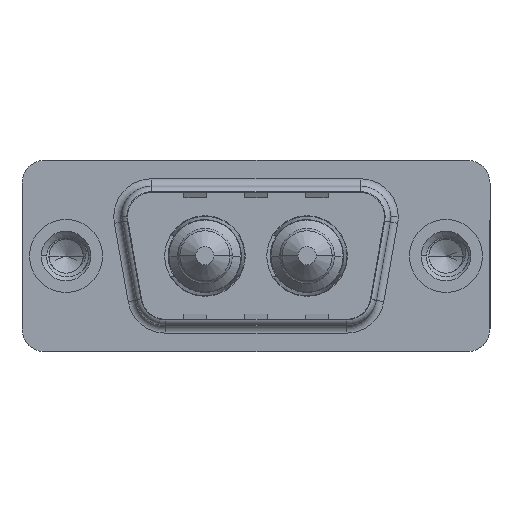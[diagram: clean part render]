
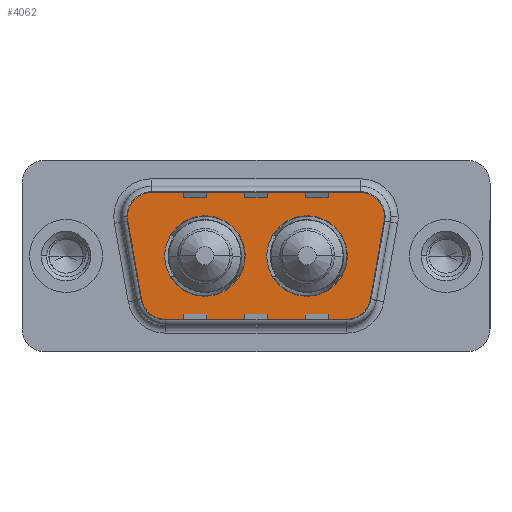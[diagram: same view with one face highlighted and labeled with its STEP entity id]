
A CAD part, top view. The second image highlights one B-rep face of the part: STEP entity #4062.
In plain terms, the highlighted planar face has unit normal (0, 0, 1).
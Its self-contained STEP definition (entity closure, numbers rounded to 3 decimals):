
#124 = DIRECTION ( 'NONE',  ( 0., 0., 1. ) ) ;
#154 = CARTESIAN_POINT ( 'NONE',  ( 4.489, -3.247, 0. ) ) ;
#207 = CARTESIAN_POINT ( 'NONE',  ( 5.436, 2.9, 0. ) ) ;
#245 = CIRCLE ( 'NONE', #4522, 2.65 ) ;
#307 = DIRECTION ( 'NONE',  ( 0., 0., 1. ) ) ;
#355 = DIRECTION ( 'NONE',  ( 0., 0., 1. ) ) ;
#426 = DIRECTION ( 'NONE',  ( -1., 0., 0. ) ) ;
#441 = DIRECTION ( 'NONE',  ( 0., 0., 1. ) ) ;
#458 = CARTESIAN_POINT ( 'NONE',  ( 9.14, 0., 0. ) ) ;
#484 = DIRECTION ( 'NONE',  ( 1., 0., 0. ) ) ;
#499 = DIRECTION ( 'NONE',  ( 1., 0., 0. ) ) ;
#538 = CARTESIAN_POINT ( 'NONE',  ( 3.466, 2.553, 0. ) ) ;
#560 = EDGE_CURVE ( 'NONE', #12153, #6827, #3407, .T. ) ;
#587 = CARTESIAN_POINT ( 'NONE',  ( 18.541, -4.9, 0. ) ) ;
#664 = DIRECTION ( 'NONE',  ( 0., 0., 1. ) ) ;
#837 = VERTEX_POINT ( 'NONE', #5940 ) ;
#878 = EDGE_CURVE ( 'NONE', #1156, #8185, #3256, .T. ) ;
#952 = EDGE_CURVE ( 'NONE', #6827, #12153, #5564, .T. ) ;
#1031 = LINE ( 'NONE', #9807, #10657 ) ;
#1056 = CARTESIAN_POINT ( 'NONE',  ( 15.86, 0., 0. ) ) ;
#1123 = VECTOR ( 'NONE', #4236, 1000. ) ;
#1156 = VERTEX_POINT ( 'NONE', #9752 ) ;
#1205 = DIRECTION ( 'NONE',  ( 1., 0., 0. ) ) ;
#1322 = ORIENTED_EDGE ( 'NONE', *, *, #3347, .F. ) ;
#1721 = LINE ( 'NONE', #3648, #1123 ) ;
#1875 = CARTESIAN_POINT ( 'NONE',  ( 18.541, -2.9, 0. ) ) ;
#1966 = ORIENTED_EDGE ( 'NONE', *, *, #2773, .T. ) ;
#2060 = EDGE_CURVE ( 'NONE', #8839, #4864, #4943, .T. ) ;
#2067 = DIRECTION ( 'NONE',  ( 1., 0., 0. ) ) ;
#2173 = FACE_BOUND ( 'NONE', #10236, .T. ) ;
#2336 = CIRCLE ( 'NONE', #7982, 2. ) ;
#2423 = VERTEX_POINT ( 'NONE', #6713 ) ;
#2604 = CARTESIAN_POINT ( 'NONE',  ( 6.459, -4.9, 0. ) ) ;
#2773 = EDGE_CURVE ( 'NONE', #5269, #12408, #7639, .T. ) ;
#2802 = ORIENTED_EDGE ( 'NONE', *, *, #5728, .T. ) ;
#2943 = AXIS2_PLACEMENT_3D ( 'NONE', #207, #441, #1205 ) ;
#3172 = EDGE_CURVE ( 'NONE', #5515, #2423, #2336, .T. ) ;
#3201 = DIRECTION ( 'NONE',  ( 1., 0., 0. ) ) ;
#3256 = CIRCLE ( 'NONE', #4818, 2. ) ;
#3347 = EDGE_CURVE ( 'NONE', #4761, #837, #245, .T. ) ;
#3407 = CIRCLE ( 'NONE', #5064, 2.65 ) ;
#3524 = AXIS2_PLACEMENT_3D ( 'NONE', #5838, #6750, #12303 ) ;
#3648 = CARTESIAN_POINT ( 'NONE',  ( 5.436, 4.9, 0. ) ) ;
#3705 = CARTESIAN_POINT ( 'NONE',  ( 6.459, -4.9, 0. ) ) ;
#3807 = LINE ( 'NONE', #5099, #5806 ) ;
#3814 = EDGE_CURVE ( 'NONE', #8185, #8839, #1721, .T. ) ;
#3886 = ORIENTED_EDGE ( 'NONE', *, *, #7821, .F. ) ;
#4062 = ADVANCED_FACE ( 'NONE', ( #4433, #2173, #6999 ), #6390, .T. ) ;
#4107 = ORIENTED_EDGE ( 'NONE', *, *, #3814, .T. ) ;
#4236 = DIRECTION ( 'NONE',  ( -1., 0., 0. ) ) ;
#4362 = CARTESIAN_POINT ( 'NONE',  ( 18.51, 0., 0. ) ) ;
#4433 = FACE_BOUND ( 'NONE', #10389, .T. ) ;
#4522 = AXIS2_PLACEMENT_3D ( 'NONE', #458, #355, #484 ) ;
#4574 = DIRECTION ( 'NONE',  ( 0.174, 0.985, 0. ) ) ;
#4695 = AXIS2_PLACEMENT_3D ( 'NONE', #1875, #664, #499 ) ;
#4761 = VERTEX_POINT ( 'NONE', #9322 ) ;
#4818 = AXIS2_PLACEMENT_3D ( 'NONE', #12176, #5378, #426 ) ;
#4864 = VERTEX_POINT ( 'NONE', #538 ) ;
#4943 = CIRCLE ( 'NONE', #2943, 2. ) ;
#5064 = AXIS2_PLACEMENT_3D ( 'NONE', #11351, #11273, #9793 ) ;
#5099 = CARTESIAN_POINT ( 'NONE',  ( 3.466, 2.553, 0. ) ) ;
#5269 = VERTEX_POINT ( 'NONE', #154 ) ;
#5378 = DIRECTION ( 'NONE',  ( 0., 0., 1. ) ) ;
#5380 = EDGE_CURVE ( 'NONE', #12408, #5515, #6913, .T. ) ;
#5515 = VERTEX_POINT ( 'NONE', #587 ) ;
#5564 = CIRCLE ( 'NONE', #7404, 2.65 ) ;
#5728 = EDGE_CURVE ( 'NONE', #2423, #7436, #1031, .T. ) ;
#5754 = CARTESIAN_POINT ( 'NONE',  ( 19.564, 4.9, 0. ) ) ;
#5806 = VECTOR ( 'NONE', #6979, 1000. ) ;
#5838 = CARTESIAN_POINT ( 'NONE',  ( 6.459, -2.9, 0. ) ) ;
#5900 = CARTESIAN_POINT ( 'NONE',  ( 19.564, 2.9, 0. ) ) ;
#5940 = CARTESIAN_POINT ( 'NONE',  ( 6.49, 0., 0. ) ) ;
#5942 = DIRECTION ( 'NONE',  ( 0., 0., 1. ) ) ;
#5987 = CARTESIAN_POINT ( 'NONE',  ( 13.21, 0., 0. ) ) ;
#6082 = CARTESIAN_POINT ( 'NONE',  ( 9.14, 0., 0. ) ) ;
#6390 = PLANE ( 'NONE',  #4695 ) ;
#6405 = CIRCLE ( 'NONE', #12018, 2. ) ;
#6713 = CARTESIAN_POINT ( 'NONE',  ( 20.511, -3.247, 0. ) ) ;
#6750 = DIRECTION ( 'NONE',  ( 0., 0., 1. ) ) ;
#6827 = VERTEX_POINT ( 'NONE', #5987 ) ;
#6842 = CARTESIAN_POINT ( 'NONE',  ( 5.436, 4.9, 0. ) ) ;
#6847 = DIRECTION ( 'NONE',  ( -1., 0., 0. ) ) ;
#6913 = LINE ( 'NONE', #2604, #9761 ) ;
#6979 = DIRECTION ( 'NONE',  ( 0.174, -0.985, 0. ) ) ;
#6999 = FACE_OUTER_BOUND ( 'NONE', #10603, .T. ) ;
#7042 = DIRECTION ( 'NONE',  ( 1., 0., 0. ) ) ;
#7235 = EDGE_CURVE ( 'NONE', #7436, #1156, #6405, .T. ) ;
#7404 = AXIS2_PLACEMENT_3D ( 'NONE', #1056, #8881, #2067 ) ;
#7436 = VERTEX_POINT ( 'NONE', #12067 ) ;
#7553 = ORIENTED_EDGE ( 'NONE', *, *, #3172, .T. ) ;
#7639 = CIRCLE ( 'NONE', #3524, 2. ) ;
#7821 = EDGE_CURVE ( 'NONE', #837, #4761, #8658, .T. ) ;
#7982 = AXIS2_PLACEMENT_3D ( 'NONE', #10172, #5942, #9683 ) ;
#8095 = ORIENTED_EDGE ( 'NONE', *, *, #7235, .T. ) ;
#8185 = VERTEX_POINT ( 'NONE', #5754 ) ;
#8316 = EDGE_CURVE ( 'NONE', #4864, #5269, #3807, .T. ) ;
#8658 = CIRCLE ( 'NONE', #11537, 2.65 ) ;
#8839 = VERTEX_POINT ( 'NONE', #6842 ) ;
#8881 = DIRECTION ( 'NONE',  ( 0., 0., 1. ) ) ;
#9286 = ORIENTED_EDGE ( 'NONE', *, *, #878, .T. ) ;
#9322 = CARTESIAN_POINT ( 'NONE',  ( 11.79, 0., 0. ) ) ;
#9683 = DIRECTION ( 'NONE',  ( 1., 0., 0. ) ) ;
#9752 = CARTESIAN_POINT ( 'NONE',  ( 21.564, 2.9, 0. ) ) ;
#9756 = ORIENTED_EDGE ( 'NONE', *, *, #560, .F. ) ;
#9761 = VECTOR ( 'NONE', #3201, 1000. ) ;
#9762 = ORIENTED_EDGE ( 'NONE', *, *, #952, .F. ) ;
#9793 = DIRECTION ( 'NONE',  ( 1., 0., 0. ) ) ;
#9807 = CARTESIAN_POINT ( 'NONE',  ( 21.534, 2.553, 0. ) ) ;
#10172 = CARTESIAN_POINT ( 'NONE',  ( 18.541, -2.9, 0. ) ) ;
#10236 = EDGE_LOOP ( 'NONE', ( #1322, #3886 ) ) ;
#10389 = EDGE_LOOP ( 'NONE', ( #9756, #9762 ) ) ;
#10603 = EDGE_LOOP ( 'NONE', ( #7553, #2802, #8095, #9286, #4107, #11430, #12282, #1966, #12331 ) ) ;
#10657 = VECTOR ( 'NONE', #4574, 1000. ) ;
#11273 = DIRECTION ( 'NONE',  ( 0., 0., 1. ) ) ;
#11351 = CARTESIAN_POINT ( 'NONE',  ( 15.86, 0., 0. ) ) ;
#11430 = ORIENTED_EDGE ( 'NONE', *, *, #2060, .T. ) ;
#11537 = AXIS2_PLACEMENT_3D ( 'NONE', #6082, #307, #7042 ) ;
#12018 = AXIS2_PLACEMENT_3D ( 'NONE', #5900, #124, #6847 ) ;
#12067 = CARTESIAN_POINT ( 'NONE',  ( 21.534, 2.553, 0. ) ) ;
#12153 = VERTEX_POINT ( 'NONE', #4362 ) ;
#12176 = CARTESIAN_POINT ( 'NONE',  ( 19.564, 2.9, 0. ) ) ;
#12282 = ORIENTED_EDGE ( 'NONE', *, *, #8316, .T. ) ;
#12303 = DIRECTION ( 'NONE',  ( -1., 0., 0. ) ) ;
#12331 = ORIENTED_EDGE ( 'NONE', *, *, #5380, .T. ) ;
#12408 = VERTEX_POINT ( 'NONE', #3705 ) ;
